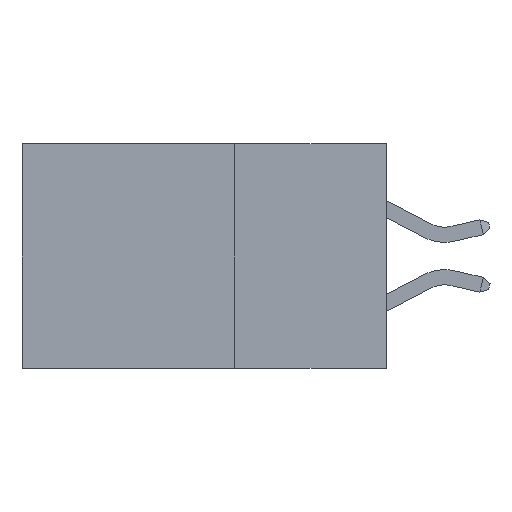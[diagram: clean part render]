
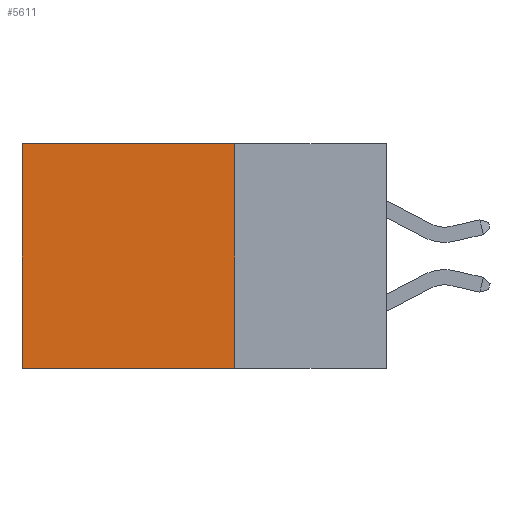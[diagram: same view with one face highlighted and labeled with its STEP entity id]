
A CAD part, left-side view. The second image highlights one B-rep face of the part: STEP entity #5611.
In plain terms, the highlighted planar face has unit normal (-1, 0, 0).
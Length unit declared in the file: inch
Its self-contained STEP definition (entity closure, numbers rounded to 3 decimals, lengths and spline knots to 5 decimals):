
#509 = DIRECTION ( 'NONE',  ( 0., 1., 0. ) ) ;
#791 = LINE ( 'NONE', #16293, #12311 ) ;
#802 = CARTESIAN_POINT ( 'NONE',  ( 0.2615, 0.25, -0.37 ) ) ;
#1341 = ORIENTED_EDGE ( 'NONE', *, *, #11196, .T. ) ;
#1620 = CARTESIAN_POINT ( 'NONE',  ( 0.2615, 0.25, 0. ) ) ;
#2183 = VECTOR ( 'NONE', #9823, 39.37008 ) ;
#2534 = VERTEX_POINT ( 'NONE', #7702 ) ;
#2965 = CARTESIAN_POINT ( 'NONE',  ( 0.2615, 0.25, -0.37 ) ) ;
#3619 = VERTEX_POINT ( 'NONE', #10814 ) ;
#4252 = FACE_OUTER_BOUND ( 'NONE', #11975, .T. ) ;
#5611 = ADVANCED_FACE ( 'NONE', ( #4252 ), #13437, .F. ) ;
#6687 = CARTESIAN_POINT ( 'NONE',  ( 0.2615, 0.6, -0.37 ) ) ;
#6796 = VERTEX_POINT ( 'NONE', #2965 ) ;
#7331 = ORIENTED_EDGE ( 'NONE', *, *, #11158, .T. ) ;
#7491 = VECTOR ( 'NONE', #11765, 39.37008 ) ;
#7702 = CARTESIAN_POINT ( 'NONE',  ( 0.2615, 0.6, -0.37 ) ) ;
#8609 = ORIENTED_EDGE ( 'NONE', *, *, #13859, .F. ) ;
#8634 = DIRECTION ( 'NONE',  ( 0., 1., 0. ) ) ;
#9823 = DIRECTION ( 'NONE',  ( 0., 0., -1. ) ) ;
#10481 = LINE ( 'NONE', #6687, #2183 ) ;
#10814 = CARTESIAN_POINT ( 'NONE',  ( 0.2615, 0.6, 0. ) ) ;
#11158 = EDGE_CURVE ( 'NONE', #3619, #2534, #10481, .T. ) ;
#11196 = EDGE_CURVE ( 'NONE', #19341, #3619, #17214, .T. ) ;
#11690 = ORIENTED_EDGE ( 'NONE', *, *, #13279, .F. ) ;
#11765 = DIRECTION ( 'NONE',  ( 0., 0., -1. ) ) ;
#11975 = EDGE_LOOP ( 'NONE', ( #7331, #11690, #8609, #1341 ) ) ;
#12311 = VECTOR ( 'NONE', #8634, 39.37008 ) ;
#13139 = VECTOR ( 'NONE', #509, 39.37008 ) ;
#13277 = DIRECTION ( 'NONE',  ( 0., 0., -1. ) ) ;
#13279 = EDGE_CURVE ( 'NONE', #6796, #2534, #791, .T. ) ;
#13330 = DIRECTION ( 'NONE',  ( 1., 0., 0. ) ) ;
#13347 = CARTESIAN_POINT ( 'NONE',  ( 0.2615, 0.25, -0.37 ) ) ;
#13437 = PLANE ( 'NONE',  #16417 ) ;
#13859 = EDGE_CURVE ( 'NONE', #19341, #6796, #15218, .T. ) ;
#15218 = LINE ( 'NONE', #802, #7491 ) ;
#16069 = CARTESIAN_POINT ( 'NONE',  ( 0.2615, 0.25, 0. ) ) ;
#16293 = CARTESIAN_POINT ( 'NONE',  ( 0.2615, 0.25, -0.37 ) ) ;
#16417 = AXIS2_PLACEMENT_3D ( 'NONE', #13347, #13330, #13277 ) ;
#17214 = LINE ( 'NONE', #16069, #13139 ) ;
#19341 = VERTEX_POINT ( 'NONE', #1620 ) ;
